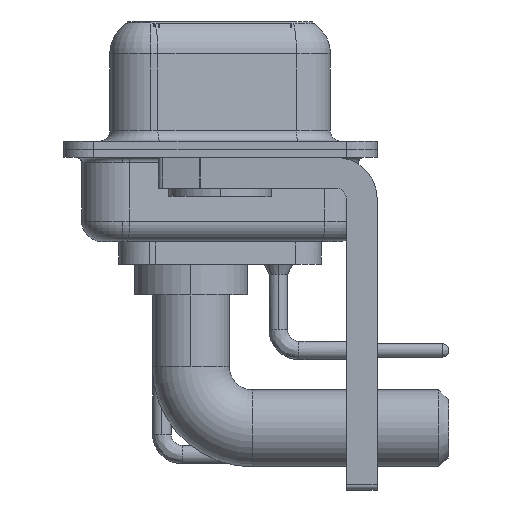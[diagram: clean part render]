
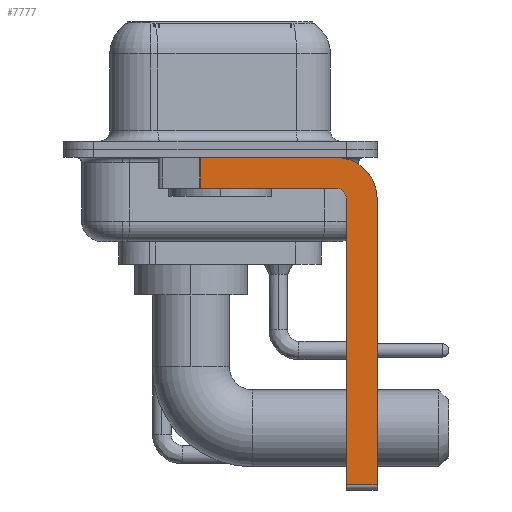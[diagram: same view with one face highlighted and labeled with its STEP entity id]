
A CAD part, left-side view. The second image highlights one B-rep face of the part: STEP entity #7777.
In plain terms, the highlighted planar face has unit normal (-1, 0, 0).
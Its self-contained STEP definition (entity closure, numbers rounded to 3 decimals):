
#1274 = DIRECTION ( 'NONE',  ( 0., 0., -1. ) ) ;
#1581 = CARTESIAN_POINT ( 'NONE',  ( -2.9, -7.65, -2.4 ) ) ;
#2822 = EDGE_LOOP ( 'NONE', ( #16423, #27959, #31151, #10287, #16793, #21854, #24976, #33041 ) ) ;
#2873 = CARTESIAN_POINT ( 'NONE',  ( -2.9, -7.65, -2.4 ) ) ;
#3156 = DIRECTION ( 'NONE',  ( 0., 0., -1. ) ) ;
#3478 = VECTOR ( 'NONE', #32233, 1000. ) ;
#3882 = CARTESIAN_POINT ( 'NONE',  ( -2.9, -5.65, -2.4 ) ) ;
#4776 = VERTEX_POINT ( 'NONE', #15696 ) ;
#5813 = VERTEX_POINT ( 'NONE', #29200 ) ;
#5834 = LINE ( 'NONE', #21155, #8031 ) ;
#6599 = AXIS2_PLACEMENT_3D ( 'NONE', #24008, #23839, #21809 ) ;
#7490 = CIRCLE ( 'NONE', #17713, 2. ) ;
#7777 = ADVANCED_FACE ( 'NONE', ( #11446 ), #21720, .F. ) ;
#8031 = VECTOR ( 'NONE', #3156, 1000. ) ;
#8635 = CARTESIAN_POINT ( 'NONE',  ( -2.9, -6.15, -16.6 ) ) ;
#8674 = VERTEX_POINT ( 'NONE', #11695 ) ;
#8779 = CARTESIAN_POINT ( 'NONE',  ( -2.9, 3., -0.4 ) ) ;
#9844 = CARTESIAN_POINT ( 'NONE',  ( -2.9, -5.65, -1.9 ) ) ;
#9867 = VERTEX_POINT ( 'NONE', #13632 ) ;
#10287 = ORIENTED_EDGE ( 'NONE', *, *, #21331, .F. ) ;
#10734 = VECTOR ( 'NONE', #30744, 1000. ) ;
#11446 = FACE_OUTER_BOUND ( 'NONE', #2822, .T. ) ;
#11496 = LINE ( 'NONE', #23628, #33006 ) ;
#11695 = CARTESIAN_POINT ( 'NONE',  ( -2.9, -6.15, -16.35 ) ) ;
#11697 = LINE ( 'NONE', #1581, #3478 ) ;
#11701 = AXIS2_PLACEMENT_3D ( 'NONE', #3882, #13492, #21889 ) ;
#13492 = DIRECTION ( 'NONE',  ( 1., 0., 0. ) ) ;
#13632 = CARTESIAN_POINT ( 'NONE',  ( -2.9, -5.65, -1.9 ) ) ;
#14095 = CARTESIAN_POINT ( 'NONE',  ( -2.9, -5.65, -2.4 ) ) ;
#15232 = CIRCLE ( 'NONE', #6599, 0.5 ) ;
#15696 = CARTESIAN_POINT ( 'NONE',  ( -2.9, 0.978, -1.9 ) ) ;
#15922 = DIRECTION ( 'NONE',  ( 0., -1., 0. ) ) ;
#16423 = ORIENTED_EDGE ( 'NONE', *, *, #23625, .F. ) ;
#16793 = ORIENTED_EDGE ( 'NONE', *, *, #21863, .F. ) ;
#17323 = EDGE_CURVE ( 'NONE', #9867, #4776, #25519, .T. ) ;
#17713 = AXIS2_PLACEMENT_3D ( 'NONE', #14095, #24360, #1274 ) ;
#18441 = VERTEX_POINT ( 'NONE', #2873 ) ;
#18678 = VERTEX_POINT ( 'NONE', #21201 ) ;
#21155 = CARTESIAN_POINT ( 'NONE',  ( -2.9, 0.978, -1.9 ) ) ;
#21201 = CARTESIAN_POINT ( 'NONE',  ( -2.9, -5.65, -0.4 ) ) ;
#21331 = EDGE_CURVE ( 'NONE', #23192, #9867, #15232, .T. ) ;
#21561 = EDGE_CURVE ( 'NONE', #18441, #22762, #11697, .T. ) ;
#21720 = PLANE ( 'NONE',  #11701 ) ;
#21733 = EDGE_CURVE ( 'NONE', #8674, #22762, #11496, .T. ) ;
#21769 = DIRECTION ( 'NONE',  ( 0., 0., 1. ) ) ;
#21809 = DIRECTION ( 'NONE',  ( 0., 0., 1. ) ) ;
#21854 = ORIENTED_EDGE ( 'NONE', *, *, #21733, .T. ) ;
#21863 = EDGE_CURVE ( 'NONE', #8674, #23192, #29377, .T. ) ;
#21889 = DIRECTION ( 'NONE',  ( 0., 0., -1. ) ) ;
#22762 = VERTEX_POINT ( 'NONE', #27219 ) ;
#23192 = VERTEX_POINT ( 'NONE', #24635 ) ;
#23625 = EDGE_CURVE ( 'NONE', #5813, #18678, #31844, .T. ) ;
#23628 = CARTESIAN_POINT ( 'NONE',  ( -2.9, -5.65, -16.35 ) ) ;
#23839 = DIRECTION ( 'NONE',  ( -1., 0., 0. ) ) ;
#23850 = VECTOR ( 'NONE', #31515, 1000. ) ;
#24008 = CARTESIAN_POINT ( 'NONE',  ( -2.9, -5.65, -2.4 ) ) ;
#24360 = DIRECTION ( 'NONE',  ( 1., 0., 0. ) ) ;
#24635 = CARTESIAN_POINT ( 'NONE',  ( -2.9, -6.15, -2.4 ) ) ;
#24976 = ORIENTED_EDGE ( 'NONE', *, *, #21561, .F. ) ;
#25519 = LINE ( 'NONE', #9844, #10734 ) ;
#27219 = CARTESIAN_POINT ( 'NONE',  ( -2.9, -7.65, -16.35 ) ) ;
#27959 = ORIENTED_EDGE ( 'NONE', *, *, #31004, .T. ) ;
#29170 = VECTOR ( 'NONE', #21769, 1000. ) ;
#29200 = CARTESIAN_POINT ( 'NONE',  ( -2.9, 0.978, -0.4 ) ) ;
#29377 = LINE ( 'NONE', #8635, #29170 ) ;
#30744 = DIRECTION ( 'NONE',  ( 0., 1., 0. ) ) ;
#31004 = EDGE_CURVE ( 'NONE', #5813, #4776, #5834, .T. ) ;
#31128 = EDGE_CURVE ( 'NONE', #18678, #18441, #7490, .T. ) ;
#31151 = ORIENTED_EDGE ( 'NONE', *, *, #17323, .F. ) ;
#31515 = DIRECTION ( 'NONE',  ( 0., -1., 0. ) ) ;
#31844 = LINE ( 'NONE', #8779, #23850 ) ;
#32233 = DIRECTION ( 'NONE',  ( 0., 0., -1. ) ) ;
#33006 = VECTOR ( 'NONE', #15922, 1000. ) ;
#33041 = ORIENTED_EDGE ( 'NONE', *, *, #31128, .F. ) ;
